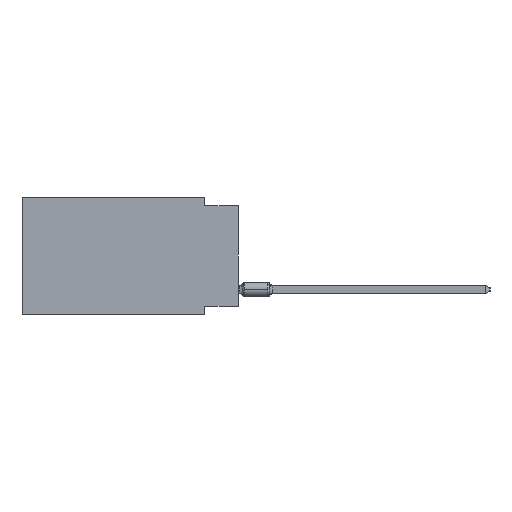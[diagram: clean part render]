
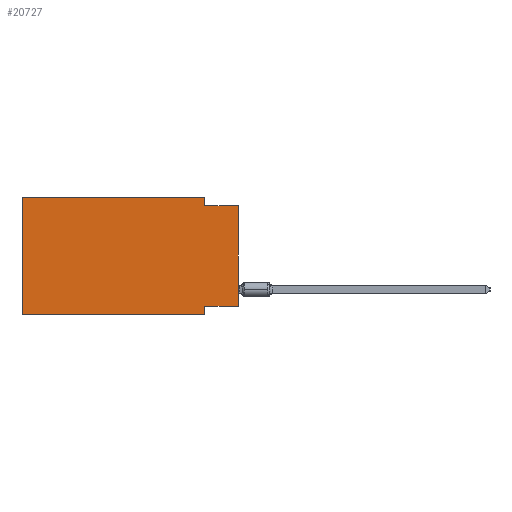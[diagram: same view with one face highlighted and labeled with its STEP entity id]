
A CAD part, left-side view. The second image highlights one B-rep face of the part: STEP entity #20727.
In plain terms, the highlighted planar face has unit normal (-1, 0, 0).
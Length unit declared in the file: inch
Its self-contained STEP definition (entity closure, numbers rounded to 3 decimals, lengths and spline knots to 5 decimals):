
#309 = CARTESIAN_POINT ( 'NONE',  ( 0., 0.1, -0.35 ) ) ;
#842 = CARTESIAN_POINT ( 'NONE',  ( 0., 0.1, -0.325 ) ) ;
#1291 = CARTESIAN_POINT ( 'NONE',  ( 0., 0.645, -0.35 ) ) ;
#1706 = LINE ( 'NONE', #28317, #15371 ) ;
#1905 = DIRECTION ( 'NONE',  ( 0., 0., -1. ) ) ;
#2053 = LINE ( 'NONE', #19471, #15700 ) ;
#2142 = CARTESIAN_POINT ( 'NONE',  ( 0., 0.1, 0. ) ) ;
#2421 = EDGE_CURVE ( 'NONE', #3813, #6399, #17528, .T. ) ;
#2696 = ORIENTED_EDGE ( 'NONE', *, *, #10532, .F. ) ;
#3509 = CARTESIAN_POINT ( 'NONE',  ( 0., 0., -0.025 ) ) ;
#3813 = VERTEX_POINT ( 'NONE', #17810 ) ;
#4558 = VERTEX_POINT ( 'NONE', #28602 ) ;
#4842 = VECTOR ( 'NONE', #27924, 39.37008 ) ;
#5315 = AXIS2_PLACEMENT_3D ( 'NONE', #15581, #24800, #19823 ) ;
#5889 = ORIENTED_EDGE ( 'NONE', *, *, #6415, .F. ) ;
#5996 = CARTESIAN_POINT ( 'NONE',  ( 0., 0.1, -0.35 ) ) ;
#6399 = VERTEX_POINT ( 'NONE', #6935 ) ;
#6415 = EDGE_CURVE ( 'NONE', #4558, #8594, #1706, .T. ) ;
#6746 = LINE ( 'NONE', #25938, #16168 ) ;
#6935 = CARTESIAN_POINT ( 'NONE',  ( 0., 0., -0.025 ) ) ;
#8568 = PLANE ( 'NONE',  #5315 ) ;
#8594 = VERTEX_POINT ( 'NONE', #842 ) ;
#9468 = LINE ( 'NONE', #22777, #28635 ) ;
#9567 = ORIENTED_EDGE ( 'NONE', *, *, #26403, .T. ) ;
#10532 = EDGE_CURVE ( 'NONE', #18448, #24433, #2053, .T. ) ;
#10980 = DIRECTION ( 'NONE',  ( 0., -1., 0. ) ) ;
#11154 = EDGE_LOOP ( 'NONE', ( #14074, #17395, #27527, #2696, #28829, #9567, #26802, #5889 ) ) ;
#12480 = LINE ( 'NONE', #16990, #13981 ) ;
#13396 = EDGE_CURVE ( 'NONE', #24433, #3813, #6746, .T. ) ;
#13981 = VECTOR ( 'NONE', #19343, 39.37008 ) ;
#14074 = ORIENTED_EDGE ( 'NONE', *, *, #22081, .T. ) ;
#14091 = EDGE_CURVE ( 'NONE', #20197, #18448, #19780, .T. ) ;
#15167 = DIRECTION ( 'NONE',  ( 0., 1., 0. ) ) ;
#15371 = VECTOR ( 'NONE', #15167, 39.37008 ) ;
#15535 = CARTESIAN_POINT ( 'NONE',  ( 0., 0.645, 0. ) ) ;
#15581 = CARTESIAN_POINT ( 'NONE',  ( 0., 0.645, 0. ) ) ;
#15700 = VECTOR ( 'NONE', #10980, 39.37008 ) ;
#16168 = VECTOR ( 'NONE', #1905, 39.37008 ) ;
#16533 = VERTEX_POINT ( 'NONE', #309 ) ;
#16990 = CARTESIAN_POINT ( 'NONE',  ( 0., 0.645, -0.35 ) ) ;
#17390 = CARTESIAN_POINT ( 'NONE',  ( 0., 0.645, 0. ) ) ;
#17395 = ORIENTED_EDGE ( 'NONE', *, *, #2421, .F. ) ;
#17528 = LINE ( 'NONE', #3509, #27133 ) ;
#17810 = CARTESIAN_POINT ( 'NONE',  ( 0., 0.1, -0.025 ) ) ;
#18448 = VERTEX_POINT ( 'NONE', #17390 ) ;
#19343 = DIRECTION ( 'NONE',  ( 0., -1., 0. ) ) ;
#19471 = CARTESIAN_POINT ( 'NONE',  ( 0., 0.645, 0. ) ) ;
#19780 = LINE ( 'NONE', #15535, #22885 ) ;
#19823 = DIRECTION ( 'NONE',  ( 0., 0., -1. ) ) ;
#20197 = VERTEX_POINT ( 'NONE', #1291 ) ;
#20727 = ADVANCED_FACE ( 'NONE', ( #28593 ), #8568, .F. ) ;
#21344 = DIRECTION ( 'NONE',  ( 0., -1., 0. ) ) ;
#22081 = EDGE_CURVE ( 'NONE', #4558, #6399, #9468, .T. ) ;
#22777 = CARTESIAN_POINT ( 'NONE',  ( 0., 0., 0. ) ) ;
#22885 = VECTOR ( 'NONE', #28706, 39.37008 ) ;
#23831 = LINE ( 'NONE', #5996, #4842 ) ;
#24433 = VERTEX_POINT ( 'NONE', #2142 ) ;
#24800 = DIRECTION ( 'NONE',  ( 1., 0., 0. ) ) ;
#25938 = CARTESIAN_POINT ( 'NONE',  ( 0., 0.1, 0. ) ) ;
#26403 = EDGE_CURVE ( 'NONE', #20197, #16533, #12480, .T. ) ;
#26802 = ORIENTED_EDGE ( 'NONE', *, *, #27997, .F. ) ;
#26868 = DIRECTION ( 'NONE',  ( 0., 0., 1. ) ) ;
#27133 = VECTOR ( 'NONE', #21344, 39.37008 ) ;
#27527 = ORIENTED_EDGE ( 'NONE', *, *, #13396, .F. ) ;
#27924 = DIRECTION ( 'NONE',  ( 0., 0., -1. ) ) ;
#27997 = EDGE_CURVE ( 'NONE', #8594, #16533, #23831, .T. ) ;
#28317 = CARTESIAN_POINT ( 'NONE',  ( 0., 0., -0.325 ) ) ;
#28593 = FACE_OUTER_BOUND ( 'NONE', #11154, .T. ) ;
#28602 = CARTESIAN_POINT ( 'NONE',  ( 0., 0., -0.325 ) ) ;
#28635 = VECTOR ( 'NONE', #26868, 39.37008 ) ;
#28706 = DIRECTION ( 'NONE',  ( 0., 0., 1. ) ) ;
#28829 = ORIENTED_EDGE ( 'NONE', *, *, #14091, .F. ) ;
